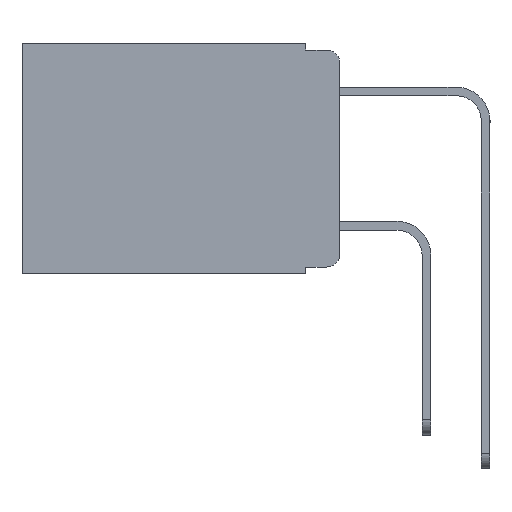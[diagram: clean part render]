
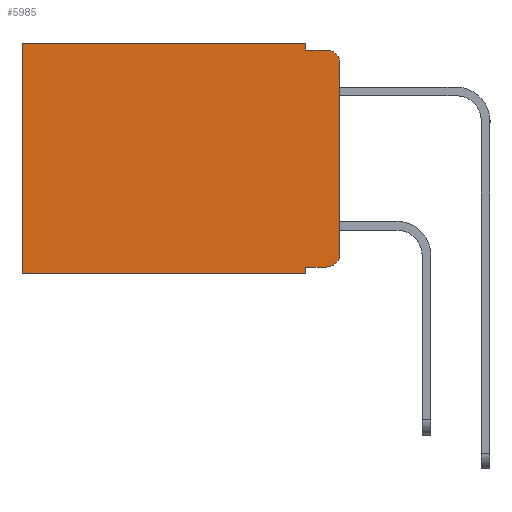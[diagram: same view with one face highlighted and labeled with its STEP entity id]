
A CAD part, left-side view. The second image highlights one B-rep face of the part: STEP entity #5985.
In plain terms, the highlighted planar face has unit normal (-1, 0, 0).
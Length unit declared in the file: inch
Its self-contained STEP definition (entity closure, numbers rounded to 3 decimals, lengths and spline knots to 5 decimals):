
#126 = VERTEX_POINT ( 'NONE', #4785 ) ;
#137 = ORIENTED_EDGE ( 'NONE', *, *, #4256, .T. ) ;
#159 = CARTESIAN_POINT ( 'NONE',  ( 0.298, 0.02, -0.333 ) ) ;
#319 = ORIENTED_EDGE ( 'NONE', *, *, #2771, .F. ) ;
#366 = CARTESIAN_POINT ( 'NONE',  ( 0.298, 0.051, -0.01 ) ) ;
#680 = VECTOR ( 'NONE', #11360, 39.37008 ) ;
#763 = ORIENTED_EDGE ( 'NONE', *, *, #2138, .F. ) ;
#1109 = ORIENTED_EDGE ( 'NONE', *, *, #1406, .T. ) ;
#1140 = AXIS2_PLACEMENT_3D ( 'NONE', #10925, #5051, #11894 ) ;
#1378 = LINE ( 'NONE', #3481, #680 ) ;
#1406 = EDGE_CURVE ( 'NONE', #11498, #7160, #4344, .T. ) ;
#1529 = VECTOR ( 'NONE', #5630, 39.37008 ) ;
#1565 = VERTEX_POINT ( 'NONE', #2495 ) ;
#2004 = DIRECTION ( 'NONE',  ( 1., 0., 0. ) ) ;
#2052 = ORIENTED_EDGE ( 'NONE', *, *, #13000, .T. ) ;
#2084 = CARTESIAN_POINT ( 'NONE',  ( 0.298, 0.051, -0.343 ) ) ;
#2088 = LINE ( 'NONE', #11514, #12048 ) ;
#2138 = EDGE_CURVE ( 'NONE', #11498, #6698, #2686, .T. ) ;
#2348 = CARTESIAN_POINT ( 'NONE',  ( 0.298, 0., 0. ) ) ;
#2388 = CARTESIAN_POINT ( 'NONE',  ( 0.298, 0.051, -0.333 ) ) ;
#2495 = CARTESIAN_POINT ( 'NONE',  ( 0.298, 0., -0.313 ) ) ;
#2686 = LINE ( 'NONE', #3199, #12871 ) ;
#2726 = DIRECTION ( 'NONE',  ( 0., 1., 0. ) ) ;
#2771 = EDGE_CURVE ( 'NONE', #6698, #5573, #3836, .T. ) ;
#3199 = CARTESIAN_POINT ( 'NONE',  ( 0.298, 0.051, 0. ) ) ;
#3362 = CARTESIAN_POINT ( 'NONE',  ( 0.298, 0.473, 0. ) ) ;
#3479 = VECTOR ( 'NONE', #12425, 39.37008 ) ;
#3481 = CARTESIAN_POINT ( 'NONE',  ( 0.298, 0.051, 0. ) ) ;
#3798 = LINE ( 'NONE', #366, #3479 ) ;
#3836 = LINE ( 'NONE', #10373, #6178 ) ;
#4125 = VECTOR ( 'NONE', #11321, 39.37008 ) ;
#4256 = EDGE_CURVE ( 'NONE', #126, #5573, #9859, .T. ) ;
#4340 = CARTESIAN_POINT ( 'NONE',  ( 0.298, 0.02, -0.03 ) ) ;
#4344 = LINE ( 'NONE', #2388, #1529 ) ;
#4374 = CIRCLE ( 'NONE', #1140, 0.02 ) ;
#4612 = VECTOR ( 'NONE', #9326, 39.37008 ) ;
#4785 = CARTESIAN_POINT ( 'NONE',  ( 0.298, 0.473, 0. ) ) ;
#4824 = AXIS2_PLACEMENT_3D ( 'NONE', #4340, #11204, #5363 ) ;
#5051 = DIRECTION ( 'NONE',  ( -1., 0., 0. ) ) ;
#5363 = DIRECTION ( 'NONE',  ( 0., 0., -1. ) ) ;
#5491 = ORIENTED_EDGE ( 'NONE', *, *, #12763, .F. ) ;
#5573 = VERTEX_POINT ( 'NONE', #12313 ) ;
#5630 = DIRECTION ( 'NONE',  ( 0., -1., 0. ) ) ;
#5764 = VERTEX_POINT ( 'NONE', #7795 ) ;
#5985 = ADVANCED_FACE ( 'NONE', ( #8421 ), #10009, .F. ) ;
#6178 = VECTOR ( 'NONE', #2726, 39.37008 ) ;
#6445 = AXIS2_PLACEMENT_3D ( 'NONE', #11941, #2004, #9060 ) ;
#6698 = VERTEX_POINT ( 'NONE', #2084 ) ;
#6937 = EDGE_CURVE ( 'NONE', #7334, #5764, #1378, .T. ) ;
#7160 = VERTEX_POINT ( 'NONE', #159 ) ;
#7334 = VERTEX_POINT ( 'NONE', #7692 ) ;
#7692 = CARTESIAN_POINT ( 'NONE',  ( 0.298, 0.051, 0. ) ) ;
#7795 = CARTESIAN_POINT ( 'NONE',  ( 0.298, 0.051, -0.01 ) ) ;
#8412 = ORIENTED_EDGE ( 'NONE', *, *, #9572, .T. ) ;
#8421 = FACE_OUTER_BOUND ( 'NONE', #12650, .T. ) ;
#8569 = CARTESIAN_POINT ( 'NONE',  ( 0.298, 0.051, -0.333 ) ) ;
#8740 = VERTEX_POINT ( 'NONE', #8885 ) ;
#8885 = CARTESIAN_POINT ( 'NONE',  ( 0.298, 0.02, -0.01 ) ) ;
#9060 = DIRECTION ( 'NONE',  ( 0., 0., -1. ) ) ;
#9207 = DIRECTION ( 'NONE',  ( 0., 0., -1. ) ) ;
#9326 = DIRECTION ( 'NONE',  ( 0., 0., -1. ) ) ;
#9572 = EDGE_CURVE ( 'NONE', #10503, #8740, #10011, .T. ) ;
#9595 = DIRECTION ( 'NONE',  ( 0., 0., -1. ) ) ;
#9659 = ORIENTED_EDGE ( 'NONE', *, *, #10848, .F. ) ;
#9859 = LINE ( 'NONE', #3362, #4612 ) ;
#10009 = PLANE ( 'NONE',  #6445 ) ;
#10011 = CIRCLE ( 'NONE', #4824, 0.02 ) ;
#10108 = EDGE_CURVE ( 'NONE', #7334, #126, #11952, .T. ) ;
#10373 = CARTESIAN_POINT ( 'NONE',  ( 0.298, 0., -0.343 ) ) ;
#10503 = VERTEX_POINT ( 'NONE', #11947 ) ;
#10848 = EDGE_CURVE ( 'NONE', #5764, #8740, #3798, .T. ) ;
#10858 = ORIENTED_EDGE ( 'NONE', *, *, #6937, .F. ) ;
#10925 = CARTESIAN_POINT ( 'NONE',  ( 0.298, 0.02, -0.313 ) ) ;
#11204 = DIRECTION ( 'NONE',  ( -1., 0., 0. ) ) ;
#11321 = DIRECTION ( 'NONE',  ( 0., 1., 0. ) ) ;
#11360 = DIRECTION ( 'NONE',  ( 0., 0., -1. ) ) ;
#11498 = VERTEX_POINT ( 'NONE', #8569 ) ;
#11514 = CARTESIAN_POINT ( 'NONE',  ( 0.298, 0., 0. ) ) ;
#11894 = DIRECTION ( 'NONE',  ( 0., 0., -1. ) ) ;
#11941 = CARTESIAN_POINT ( 'NONE',  ( 0.298, 0., 0. ) ) ;
#11947 = CARTESIAN_POINT ( 'NONE',  ( 0.298, 0., -0.03 ) ) ;
#11952 = LINE ( 'NONE', #2348, #4125 ) ;
#12048 = VECTOR ( 'NONE', #9595, 39.37008 ) ;
#12067 = ORIENTED_EDGE ( 'NONE', *, *, #10108, .T. ) ;
#12313 = CARTESIAN_POINT ( 'NONE',  ( 0.298, 0.473, -0.343 ) ) ;
#12425 = DIRECTION ( 'NONE',  ( 0., -1., 0. ) ) ;
#12650 = EDGE_LOOP ( 'NONE', ( #5491, #8412, #9659, #10858, #12067, #137, #319, #763, #1109, #2052 ) ) ;
#12763 = EDGE_CURVE ( 'NONE', #10503, #1565, #2088, .T. ) ;
#12871 = VECTOR ( 'NONE', #9207, 39.37008 ) ;
#13000 = EDGE_CURVE ( 'NONE', #7160, #1565, #4374, .T. ) ;
